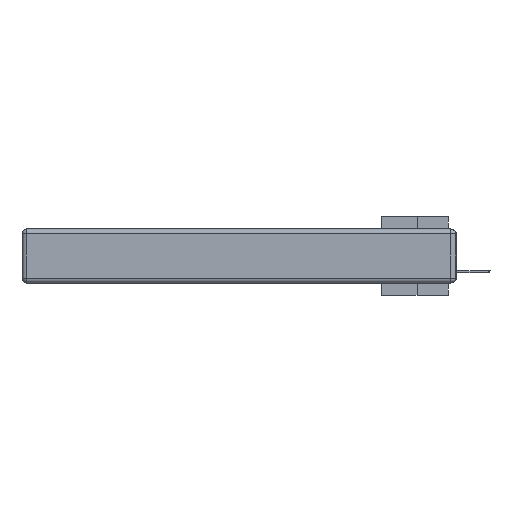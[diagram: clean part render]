
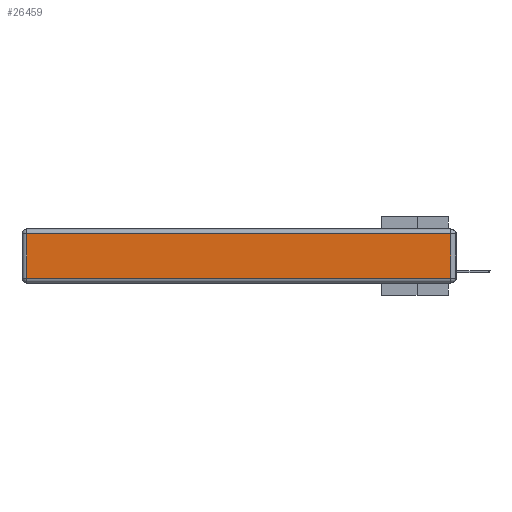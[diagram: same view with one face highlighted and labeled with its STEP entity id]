
A CAD part, left-side view. The second image highlights one B-rep face of the part: STEP entity #26459.
In plain terms, the highlighted planar face has unit normal (-1, 0, 0).
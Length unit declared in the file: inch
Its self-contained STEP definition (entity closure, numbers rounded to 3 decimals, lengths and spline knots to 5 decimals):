
#927 = EDGE_CURVE ( 'NONE', #17355, #23928, #8758, .T. ) ;
#1283 = ORIENTED_EDGE ( 'NONE', *, *, #11907, .T. ) ;
#1330 = AXIS2_PLACEMENT_3D ( 'NONE', #27877, #17628, #23154 ) ;
#1687 = CARTESIAN_POINT ( 'NONE',  ( 0., 2.72, -0.343 ) ) ;
#2014 = VECTOR ( 'NONE', #17095, 39.37008 ) ;
#3853 = PLANE ( 'NONE',  #1330 ) ;
#3875 = DIRECTION ( 'NONE',  ( 0., 1., 0. ) ) ;
#4102 = VECTOR ( 'NONE', #21194, 39.37008 ) ;
#4656 = VERTEX_POINT ( 'NONE', #5634 ) ;
#5634 = CARTESIAN_POINT ( 'NONE',  ( 0., 0.03, -0.03 ) ) ;
#6182 = LINE ( 'NONE', #8490, #14587 ) ;
#6791 = ORIENTED_EDGE ( 'NONE', *, *, #17148, .T. ) ;
#6894 = DIRECTION ( 'NONE',  ( 0., -1., 0. ) ) ;
#7796 = ORIENTED_EDGE ( 'NONE', *, *, #19661, .T. ) ;
#8118 = CARTESIAN_POINT ( 'NONE',  ( 0., 0.03, -0.343 ) ) ;
#8490 = CARTESIAN_POINT ( 'NONE',  ( 0., 2.75, -0.03 ) ) ;
#8758 = LINE ( 'NONE', #17527, #18441 ) ;
#9640 = EDGE_LOOP ( 'NONE', ( #14908, #7796, #6791, #1283 ) ) ;
#10204 = FACE_OUTER_BOUND ( 'NONE', #9640, .T. ) ;
#11907 = EDGE_CURVE ( 'NONE', #25600, #17355, #23721, .T. ) ;
#14587 = VECTOR ( 'NONE', #3875, 39.37008 ) ;
#14908 = ORIENTED_EDGE ( 'NONE', *, *, #927, .T. ) ;
#16185 = LINE ( 'NONE', #8118, #4102 ) ;
#17095 = DIRECTION ( 'NONE',  ( 0., 0., -1. ) ) ;
#17148 = EDGE_CURVE ( 'NONE', #4656, #25600, #6182, .T. ) ;
#17355 = VERTEX_POINT ( 'NONE', #24432 ) ;
#17527 = CARTESIAN_POINT ( 'NONE',  ( 0., 0., -0.313 ) ) ;
#17628 = DIRECTION ( 'NONE',  ( -1., 0., 0. ) ) ;
#18441 = VECTOR ( 'NONE', #6894, 39.37008 ) ;
#19661 = EDGE_CURVE ( 'NONE', #23928, #4656, #16185, .T. ) ;
#21194 = DIRECTION ( 'NONE',  ( 0., 0., 1. ) ) ;
#21480 = CARTESIAN_POINT ( 'NONE',  ( 0., 2.72, -0.03 ) ) ;
#23154 = DIRECTION ( 'NONE',  ( 0., 0., 1. ) ) ;
#23245 = CARTESIAN_POINT ( 'NONE',  ( 0., 0.03, -0.313 ) ) ;
#23721 = LINE ( 'NONE', #1687, #2014 ) ;
#23928 = VERTEX_POINT ( 'NONE', #23245 ) ;
#24432 = CARTESIAN_POINT ( 'NONE',  ( 0., 2.72, -0.313 ) ) ;
#25600 = VERTEX_POINT ( 'NONE', #21480 ) ;
#26459 = ADVANCED_FACE ( 'NONE', ( #10204 ), #3853, .T. ) ;
#27877 = CARTESIAN_POINT ( 'NONE',  ( 0., 0., -0.343 ) ) ;
